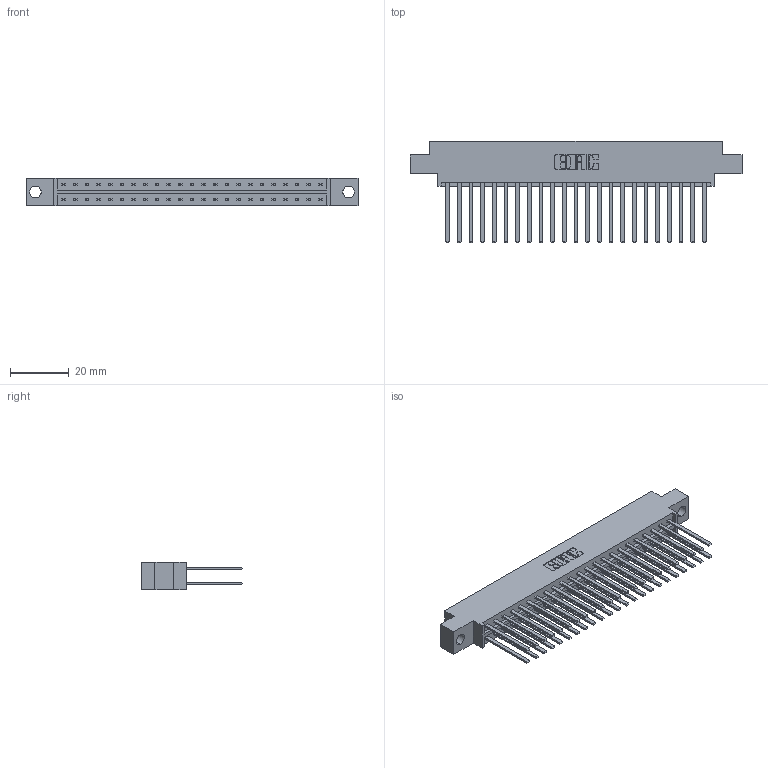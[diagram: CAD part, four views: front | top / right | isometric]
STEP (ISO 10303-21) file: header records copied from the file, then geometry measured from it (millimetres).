
FILE_DESCRIPTION (( 'STEP AP203' ), '1' );
FILE_NAME ('833-046-544-804.STEP', '2020-06-04T14:41:22', ( '' ), ( '' ), 'SwSTEP 2.0', 'SolidWorks 2020', '' );
FILE_SCHEMA (( 'CONFIG_CONTROL_DESIGN' ));
Length unit declared in the file: inch
Products named in the file (3): 833 Part_Offset - .156 Dia - TH; 833-046-544-804; 345-292-001_345-293-144
Assembly tree (47 placements, depth 2):
  833-046-544-804
    833 Part_Offset - .156 Dia - TH
    345-292-001_345-293-144  x46
Bounding box: 112.67 x 34.3 x 9.4 mm (x, y, z)
Volume: 11654.9 mm3; surface area: 15671.3 mm2
Topology: 47 solids, 47 shells, 2234 faces, 6625 edges, 4354 vertices
Faces by surface type: plane 1546, cylinder 688
Entity records: 17205 total; most frequent: CARTESIAN_POINT 2874, ORIENTED_EDGE 2810, DIRECTION 2485, EDGE_CURVE 1405, VECTOR 1281, LINE 1281, VERTEX_POINT 934, AXIS2_PLACEMENT_3D 602
